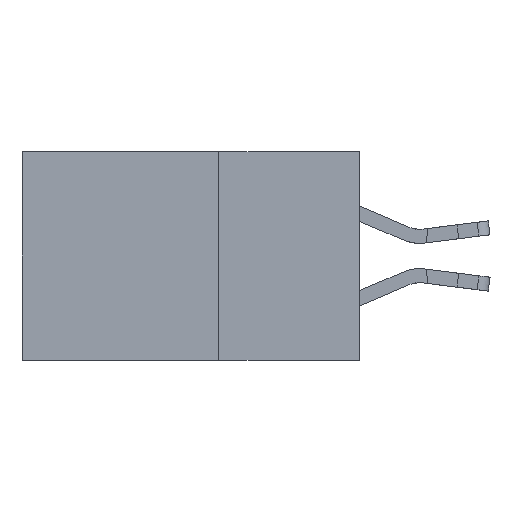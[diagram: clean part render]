
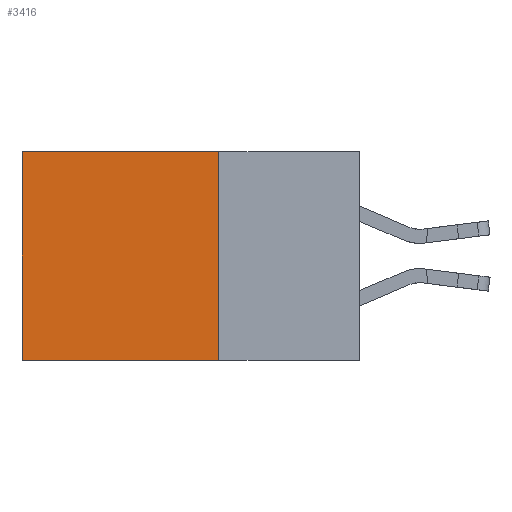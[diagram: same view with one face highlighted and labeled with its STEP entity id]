
A CAD part, left-side view. The second image highlights one B-rep face of the part: STEP entity #3416.
In plain terms, the highlighted planar face has unit normal (-1, 0, 0).
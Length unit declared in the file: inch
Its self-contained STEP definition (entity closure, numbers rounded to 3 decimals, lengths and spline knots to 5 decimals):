
#1349 = ORIENTED_EDGE ( 'NONE', *, *, #25494, .F. ) ;
#1762 = LINE ( 'NONE', #24108, #6960 ) ;
#2729 = CARTESIAN_POINT ( 'NONE',  ( 0.2875, 0.25, 0. ) ) ;
#2767 = VECTOR ( 'NONE', #13329, 39.37008 ) ;
#2778 = CARTESIAN_POINT ( 'NONE',  ( 0.2875, 0.25, 0. ) ) ;
#3416 = ADVANCED_FACE ( 'NONE', ( #29851 ), #12018, .F. ) ;
#4184 = CARTESIAN_POINT ( 'NONE',  ( 0.2875, 0.6, 0. ) ) ;
#4199 = CARTESIAN_POINT ( 'NONE',  ( 0.2875, 0.25, -0.37 ) ) ;
#4903 = EDGE_CURVE ( 'NONE', #6839, #28262, #16891, .T. ) ;
#6839 = VERTEX_POINT ( 'NONE', #4184 ) ;
#6960 = VECTOR ( 'NONE', #14791, 39.37008 ) ;
#7941 = CARTESIAN_POINT ( 'NONE',  ( 0.2875, 0.6, 0. ) ) ;
#8729 = VECTOR ( 'NONE', #10680, 39.37008 ) ;
#10452 = ORIENTED_EDGE ( 'NONE', *, *, #4903, .T. ) ;
#10680 = DIRECTION ( 'NONE',  ( 0., 0., -1. ) ) ;
#12018 = PLANE ( 'NONE',  #26070 ) ;
#12315 = DIRECTION ( 'NONE',  ( 0., 0., -1. ) ) ;
#12505 = DIRECTION ( 'NONE',  ( 1., 0., 0. ) ) ;
#12622 = DIRECTION ( 'NONE',  ( 0., 1., 0. ) ) ;
#13329 = DIRECTION ( 'NONE',  ( 0., 1., 0. ) ) ;
#14241 = EDGE_CURVE ( 'NONE', #24830, #28262, #16506, .T. ) ;
#14791 = DIRECTION ( 'NONE',  ( 0., 0., -1. ) ) ;
#16506 = LINE ( 'NONE', #4199, #2767 ) ;
#16891 = LINE ( 'NONE', #7941, #8729 ) ;
#17076 = CARTESIAN_POINT ( 'NONE',  ( 0.2875, 0.25, -0.37 ) ) ;
#19069 = VECTOR ( 'NONE', #12622, 39.37008 ) ;
#21445 = ORIENTED_EDGE ( 'NONE', *, *, #14241, .F. ) ;
#22458 = EDGE_CURVE ( 'NONE', #27828, #6839, #25013, .T. ) ;
#22913 = ORIENTED_EDGE ( 'NONE', *, *, #22458, .T. ) ;
#24108 = CARTESIAN_POINT ( 'NONE',  ( 0.2875, 0.25, 0. ) ) ;
#24267 = CARTESIAN_POINT ( 'NONE',  ( 0.2875, 0.6, -0.37 ) ) ;
#24830 = VERTEX_POINT ( 'NONE', #17076 ) ;
#25013 = LINE ( 'NONE', #2778, #19069 ) ;
#25494 = EDGE_CURVE ( 'NONE', #27828, #24830, #1762, .T. ) ;
#26070 = AXIS2_PLACEMENT_3D ( 'NONE', #26366, #12505, #12315 ) ;
#26366 = CARTESIAN_POINT ( 'NONE',  ( 0.2875, 0.25, 0. ) ) ;
#27828 = VERTEX_POINT ( 'NONE', #2729 ) ;
#28262 = VERTEX_POINT ( 'NONE', #24267 ) ;
#29851 = FACE_OUTER_BOUND ( 'NONE', #30403, .T. ) ;
#30403 = EDGE_LOOP ( 'NONE', ( #10452, #21445, #1349, #22913 ) ) ;
